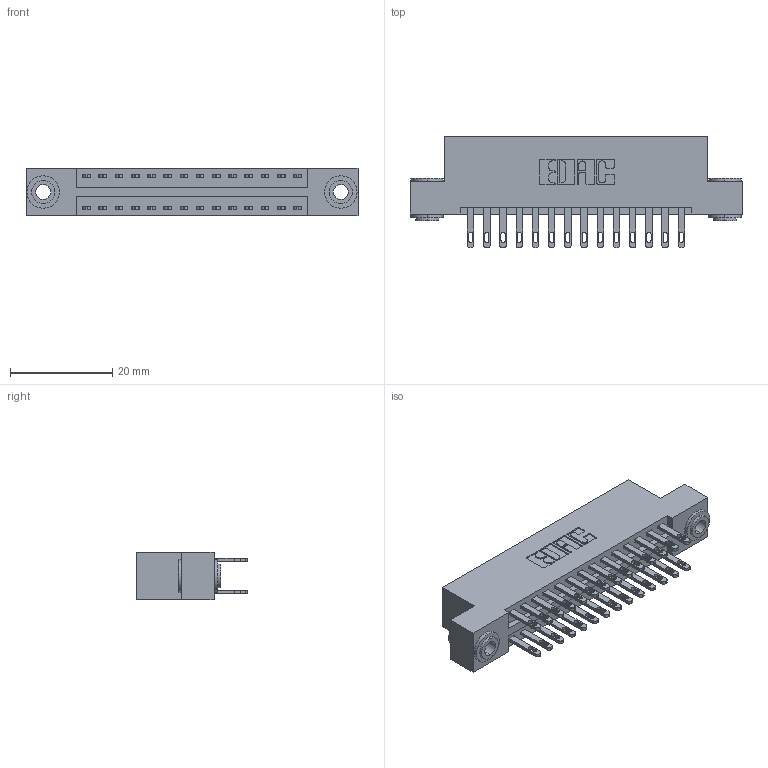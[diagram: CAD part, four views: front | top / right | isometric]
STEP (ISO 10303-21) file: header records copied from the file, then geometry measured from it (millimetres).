
FILE_DESCRIPTION (( 'STEP AP203' ), '1' );
FILE_NAME ('896-028-500-203.STEP', '2021-07-27T18:19:37', ( '' ), ( '' ), 'SwSTEP 2.0', 'SolidWorks 2020', '' );
FILE_SCHEMA (( 'CONFIG_CONTROL_DESIGN' ));
Length unit declared in the file: inch
Products named in the file (4): 896-028-500-203; 345-250-002_345-250-002-102; 846 Part_Flush Mounting Lugs - 0.156 Dia-TH; 345-292-001_345-293-100
Assembly tree (31 placements, depth 2):
  896-028-500-203
    846 Part_Flush Mounting Lugs - 0.156 Dia-TH
    345-292-001_345-293-100  x28
    345-250-002_345-250-002-102  x2
Bounding box: 65.02 x 21.84 x 9.4 mm (x, y, z)
Volume: 6228.1 mm3; surface area: 8628.1 mm2
Topology: 31 solids, 31 shells, 1504 faces, 4521 edges, 3010 vertices
Faces by surface type: plane 898, cylinder 598, cone 8
Entity records: 13486 total; most frequent: CARTESIAN_POINT 2235, ORIENTED_EDGE 2162, DIRECTION 2055, EDGE_CURVE 1081, LINE 865, VECTOR 865, VERTEX_POINT 718, AXIS2_PLACEMENT_3D 595
